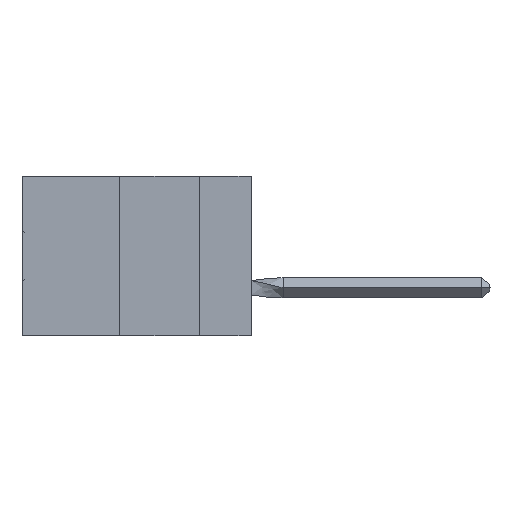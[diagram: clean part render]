
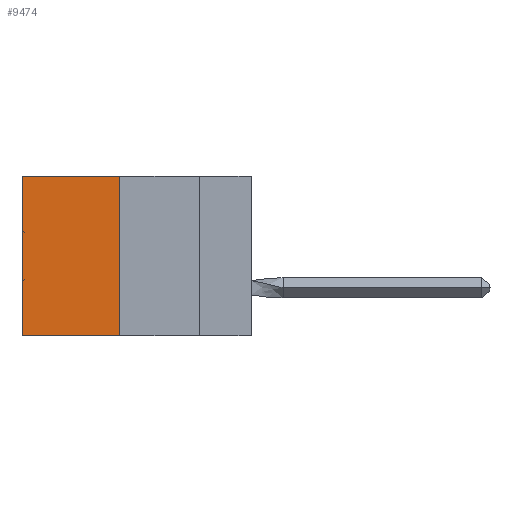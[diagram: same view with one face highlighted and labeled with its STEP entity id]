
A CAD part, left-side view. The second image highlights one B-rep face of the part: STEP entity #9474.
In plain terms, the highlighted planar face has unit normal (-1, 0, 0).
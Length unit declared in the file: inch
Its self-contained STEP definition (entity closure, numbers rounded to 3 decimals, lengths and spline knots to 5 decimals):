
#5270 = EDGE_CURVE ( 'NONE', #10399, #34558, #29577, .T. ) ;
#5772 = CARTESIAN_POINT ( 'NONE',  ( 0.305, 0.413, 0. ) ) ;
#7535 = DIRECTION ( 'NONE',  ( 0., 1., 0. ) ) ;
#9474 = ADVANCED_FACE ( 'NONE', ( #31875 ), #10604, .F. ) ;
#9978 = CARTESIAN_POINT ( 'NONE',  ( 0.305, 0.413, -0.5 ) ) ;
#10399 = VERTEX_POINT ( 'NONE', #5772 ) ;
#10604 = PLANE ( 'NONE',  #41093 ) ;
#16027 = DIRECTION ( 'NONE',  ( 0., 0., -1. ) ) ;
#16238 = VERTEX_POINT ( 'NONE', #42504 ) ;
#20382 = VECTOR ( 'NONE', #7535, 39.37008 ) ;
#21029 = LINE ( 'NONE', #33944, #27073 ) ;
#27073 = VECTOR ( 'NONE', #46344, 39.37008 ) ;
#27462 = ORIENTED_EDGE ( 'NONE', *, *, #33527, .F. ) ;
#27503 = ORIENTED_EDGE ( 'NONE', *, *, #5270, .F. ) ;
#27975 = EDGE_CURVE ( 'NONE', #10399, #16238, #21029, .T. ) ;
#29577 = LINE ( 'NONE', #9978, #53142 ) ;
#29971 = VERTEX_POINT ( 'NONE', #49724 ) ;
#31657 = LINE ( 'NONE', #41190, #45144 ) ;
#31875 = FACE_OUTER_BOUND ( 'NONE', #36966, .T. ) ;
#32525 = CARTESIAN_POINT ( 'NONE',  ( 0.305, 0.413, -0.5 ) ) ;
#33527 = EDGE_CURVE ( 'NONE', #34558, #29971, #48653, .T. ) ;
#33944 = CARTESIAN_POINT ( 'NONE',  ( 0.305, 0.413, 0. ) ) ;
#34074 = ORIENTED_EDGE ( 'NONE', *, *, #27975, .T. ) ;
#34249 = CARTESIAN_POINT ( 'NONE',  ( 0.305, 0.413, -0.5 ) ) ;
#34558 = VERTEX_POINT ( 'NONE', #34249 ) ;
#36076 = DIRECTION ( 'NONE',  ( 1., 0., 0. ) ) ;
#36966 = EDGE_LOOP ( 'NONE', ( #50537, #27462, #27503, #34074 ) ) ;
#39940 = DIRECTION ( 'NONE',  ( 0., 0., -1. ) ) ;
#41093 = AXIS2_PLACEMENT_3D ( 'NONE', #53605, #36076, #16027 ) ;
#41190 = CARTESIAN_POINT ( 'NONE',  ( 0.305, 0.72, -0.5 ) ) ;
#41562 = DIRECTION ( 'NONE',  ( 0., 0., -1. ) ) ;
#42504 = CARTESIAN_POINT ( 'NONE',  ( 0.305, 0.72, 0. ) ) ;
#45144 = VECTOR ( 'NONE', #41562, 39.37008 ) ;
#45377 = EDGE_CURVE ( 'NONE', #16238, #29971, #31657, .T. ) ;
#46344 = DIRECTION ( 'NONE',  ( 0., 1., 0. ) ) ;
#48653 = LINE ( 'NONE', #32525, #20382 ) ;
#49724 = CARTESIAN_POINT ( 'NONE',  ( 0.305, 0.72, -0.5 ) ) ;
#50537 = ORIENTED_EDGE ( 'NONE', *, *, #45377, .T. ) ;
#53142 = VECTOR ( 'NONE', #39940, 39.37008 ) ;
#53605 = CARTESIAN_POINT ( 'NONE',  ( 0.305, 0.413, -0.5 ) ) ;
